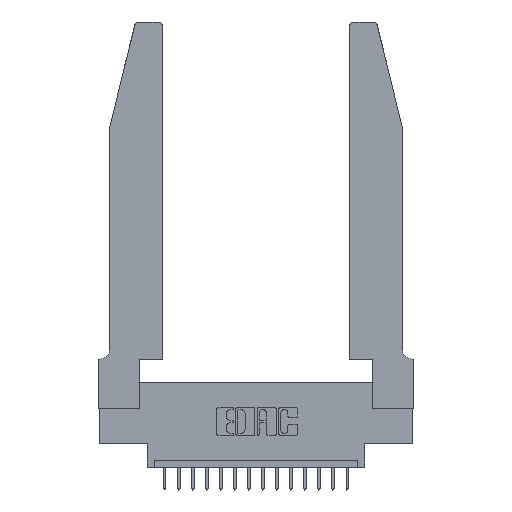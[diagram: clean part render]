
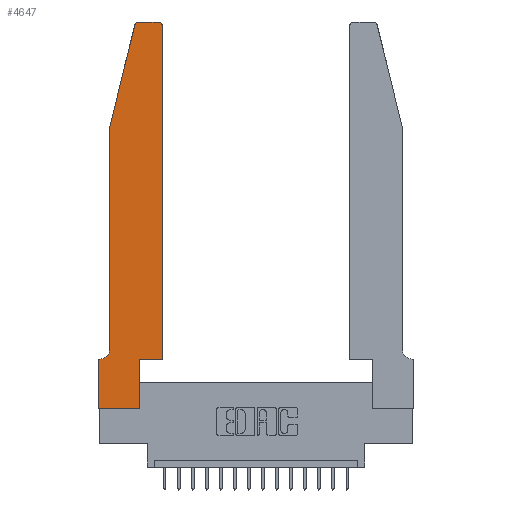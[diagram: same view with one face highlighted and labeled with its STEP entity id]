
A CAD part, top view. The second image highlights one B-rep face of the part: STEP entity #4647.
In plain terms, the highlighted planar face has unit normal (0, 0, 1).
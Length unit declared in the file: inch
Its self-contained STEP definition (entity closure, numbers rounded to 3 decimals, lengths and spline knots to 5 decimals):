
#227 = CARTESIAN_POINT ( 'NONE',  ( 0.2605, 2.75, 0.37 ) ) ;
#353 = DIRECTION ( 'NONE',  ( 0., 0., 1. ) ) ;
#615 = CARTESIAN_POINT ( 'NONE',  ( 0.0755, 2., 0.37 ) ) ;
#648 = LINE ( 'NONE', #4370, #10200 ) ;
#800 = CARTESIAN_POINT ( 'NONE',  ( 0.4205, 2.72, 0.37 ) ) ;
#839 = CARTESIAN_POINT ( 'NONE',  ( 0.2865, 0., 0.37 ) ) ;
#916 = LINE ( 'NONE', #2908, #7663 ) ;
#1175 = ORIENTED_EDGE ( 'NONE', *, *, #17467, .T. ) ;
#1439 = CARTESIAN_POINT ( 'NONE',  ( 0.0055, 0.42, 0.37 ) ) ;
#1799 = CARTESIAN_POINT ( 'NONE',  ( 0.4205, 2.75, 0.37 ) ) ;
#1901 = AXIS2_PLACEMENT_3D ( 'NONE', #1439, #13499, #13371 ) ;
#2187 = VECTOR ( 'NONE', #17022, 39.37008 ) ;
#2280 = CARTESIAN_POINT ( 'NONE',  ( 0.4505, 0.35, 0.37 ) ) ;
#2350 = VECTOR ( 'NONE', #7106, 39.37008 ) ;
#2368 = EDGE_CURVE ( 'NONE', #6960, #15596, #5971, .T. ) ;
#2398 = CARTESIAN_POINT ( 'NONE',  ( 0., 0., 0.37 ) ) ;
#2676 = CARTESIAN_POINT ( 'NONE',  ( 0., 0., 0.37 ) ) ;
#2908 = CARTESIAN_POINT ( 'NONE',  ( 0.0755, 0.35, 0.37 ) ) ;
#3000 = DIRECTION ( 'NONE',  ( -1., 0., 0. ) ) ;
#3054 = EDGE_CURVE ( 'NONE', #6041, #6938, #648, .T. ) ;
#3119 = CARTESIAN_POINT ( 'NONE',  ( 0.0055, 0.35, 0.37 ) ) ;
#3195 = ORIENTED_EDGE ( 'NONE', *, *, #6051, .T. ) ;
#3302 = EDGE_LOOP ( 'NONE', ( #6304, #18392, #19031, #18084, #15435, #14010, #3510, #1175, #16175, #15509, #3195, #8681 ) ) ;
#3510 = ORIENTED_EDGE ( 'NONE', *, *, #10936, .T. ) ;
#3532 = CIRCLE ( 'NONE', #9237, 0.03 ) ;
#4081 = LINE ( 'NONE', #227, #5000 ) ;
#4370 = CARTESIAN_POINT ( 'NONE',  ( 0.2865, 0.35, 0.37 ) ) ;
#4647 = ADVANCED_FACE ( 'NONE', ( #14127 ), #18386, .T. ) ;
#4901 = EDGE_CURVE ( 'NONE', #13022, #15820, #14335, .T. ) ;
#5000 = VECTOR ( 'NONE', #3000, 39.37008 ) ;
#5220 = EDGE_CURVE ( 'NONE', #15044, #8485, #16657, .T. ) ;
#5639 = CARTESIAN_POINT ( 'NONE',  ( 0., 0.35, 0.37 ) ) ;
#5971 = CIRCLE ( 'NONE', #1901, 0.07 ) ;
#6041 = VERTEX_POINT ( 'NONE', #839 ) ;
#6051 = EDGE_CURVE ( 'NONE', #16376, #15044, #14303, .T. ) ;
#6304 = ORIENTED_EDGE ( 'NONE', *, *, #8697, .T. ) ;
#6305 = CARTESIAN_POINT ( 'NONE',  ( 0., 0., 0.37 ) ) ;
#6938 = VERTEX_POINT ( 'NONE', #16033 ) ;
#6960 = VERTEX_POINT ( 'NONE', #16052 ) ;
#7106 = DIRECTION ( 'NONE',  ( 0., -1., 0. ) ) ;
#7112 = LINE ( 'NONE', #6305, #11116 ) ;
#7527 = AXIS2_PLACEMENT_3D ( 'NONE', #11034, #18574, #8084 ) ;
#7663 = VECTOR ( 'NONE', #19076, 39.37008 ) ;
#7969 = CARTESIAN_POINT ( 'NONE',  ( 0.4505, 2.72, 0.37 ) ) ;
#8084 = DIRECTION ( 'NONE',  ( 1., 0., 0. ) ) ;
#8188 = VERTEX_POINT ( 'NONE', #13146 ) ;
#8485 = VERTEX_POINT ( 'NONE', #1799 ) ;
#8681 = ORIENTED_EDGE ( 'NONE', *, *, #5220, .T. ) ;
#8697 = EDGE_CURVE ( 'NONE', #8485, #8188, #4081, .T. ) ;
#9237 = AXIS2_PLACEMENT_3D ( 'NONE', #9375, #353, #18267 ) ;
#9375 = CARTESIAN_POINT ( 'NONE',  ( 0.284, 2.72, 0.37 ) ) ;
#9464 = EDGE_CURVE ( 'NONE', #15820, #6960, #15261, .T. ) ;
#9778 = LINE ( 'NONE', #2676, #2350 ) ;
#9790 = DIRECTION ( 'NONE',  ( -0.239, -0.971, 0. ) ) ;
#9836 = DIRECTION ( 'NONE',  ( 0., 0., 1. ) ) ;
#10140 = CARTESIAN_POINT ( 'NONE',  ( 0.25487, 2.72718, 0.37 ) ) ;
#10185 = DIRECTION ( 'NONE',  ( 1., 0., 0. ) ) ;
#10200 = VECTOR ( 'NONE', #16294, 39.37008 ) ;
#10569 = EDGE_CURVE ( 'NONE', #8188, #13022, #3532, .T. ) ;
#10936 = EDGE_CURVE ( 'NONE', #16565, #15085, #9778, .T. ) ;
#11034 = CARTESIAN_POINT ( 'NONE',  ( 0., 0.35, 0.37 ) ) ;
#11039 = CARTESIAN_POINT ( 'NONE',  ( 0.0755, 2., 0.37 ) ) ;
#11116 = VECTOR ( 'NONE', #18380, 39.37008 ) ;
#11229 = DIRECTION ( 'NONE',  ( 1., 0., 0. ) ) ;
#12214 = AXIS2_PLACEMENT_3D ( 'NONE', #800, #9836, #11229 ) ;
#12728 = VECTOR ( 'NONE', #10185, 39.37008 ) ;
#13022 = VERTEX_POINT ( 'NONE', #10140 ) ;
#13146 = CARTESIAN_POINT ( 'NONE',  ( 0.284, 2.75, 0.37 ) ) ;
#13371 = DIRECTION ( 'NONE',  ( -1., 0., 0. ) ) ;
#13413 = CARTESIAN_POINT ( 'NONE',  ( 0.4505, 0.35, 0.37 ) ) ;
#13426 = LINE ( 'NONE', #13413, #12728 ) ;
#13499 = DIRECTION ( 'NONE',  ( 0., 0., -1. ) ) ;
#14010 = ORIENTED_EDGE ( 'NONE', *, *, #15993, .T. ) ;
#14127 = FACE_OUTER_BOUND ( 'NONE', #3302, .T. ) ;
#14272 = CARTESIAN_POINT ( 'NONE',  ( 0.0755, 2., 0.37 ) ) ;
#14303 = LINE ( 'NONE', #2280, #18456 ) ;
#14335 = LINE ( 'NONE', #14272, #17340 ) ;
#14372 = DIRECTION ( 'NONE',  ( 0., 1., 0. ) ) ;
#15044 = VERTEX_POINT ( 'NONE', #7969 ) ;
#15085 = VERTEX_POINT ( 'NONE', #2398 ) ;
#15261 = LINE ( 'NONE', #11039, #2187 ) ;
#15435 = ORIENTED_EDGE ( 'NONE', *, *, #2368, .T. ) ;
#15509 = ORIENTED_EDGE ( 'NONE', *, *, #18822, .T. ) ;
#15596 = VERTEX_POINT ( 'NONE', #3119 ) ;
#15820 = VERTEX_POINT ( 'NONE', #615 ) ;
#15993 = EDGE_CURVE ( 'NONE', #15596, #16565, #916, .T. ) ;
#16033 = CARTESIAN_POINT ( 'NONE',  ( 0.2865, 0.35, 0.37 ) ) ;
#16052 = CARTESIAN_POINT ( 'NONE',  ( 0.0755, 0.42, 0.37 ) ) ;
#16175 = ORIENTED_EDGE ( 'NONE', *, *, #3054, .T. ) ;
#16294 = DIRECTION ( 'NONE',  ( 0., 1., 0. ) ) ;
#16376 = VERTEX_POINT ( 'NONE', #16994 ) ;
#16565 = VERTEX_POINT ( 'NONE', #5639 ) ;
#16657 = CIRCLE ( 'NONE', #12214, 0.03 ) ;
#16994 = CARTESIAN_POINT ( 'NONE',  ( 0.4505, 0.35, 0.37 ) ) ;
#17022 = DIRECTION ( 'NONE',  ( 0., -1., 0. ) ) ;
#17340 = VECTOR ( 'NONE', #9790, 39.37008 ) ;
#17467 = EDGE_CURVE ( 'NONE', #15085, #6041, #7112, .T. ) ;
#18084 = ORIENTED_EDGE ( 'NONE', *, *, #9464, .T. ) ;
#18267 = DIRECTION ( 'NONE',  ( 1., 0., 0. ) ) ;
#18380 = DIRECTION ( 'NONE',  ( 1., 0., 0. ) ) ;
#18386 = PLANE ( 'NONE',  #7527 ) ;
#18392 = ORIENTED_EDGE ( 'NONE', *, *, #10569, .T. ) ;
#18456 = VECTOR ( 'NONE', #14372, 39.37008 ) ;
#18574 = DIRECTION ( 'NONE',  ( 0., 0., 1. ) ) ;
#18822 = EDGE_CURVE ( 'NONE', #6938, #16376, #13426, .T. ) ;
#19031 = ORIENTED_EDGE ( 'NONE', *, *, #4901, .T. ) ;
#19076 = DIRECTION ( 'NONE',  ( -1., 0., 0. ) ) ;
